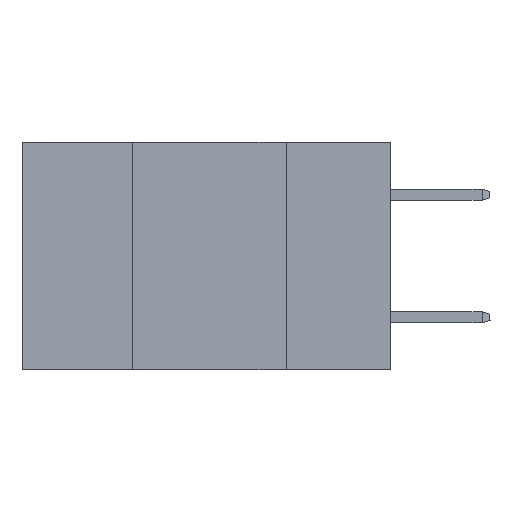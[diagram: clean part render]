
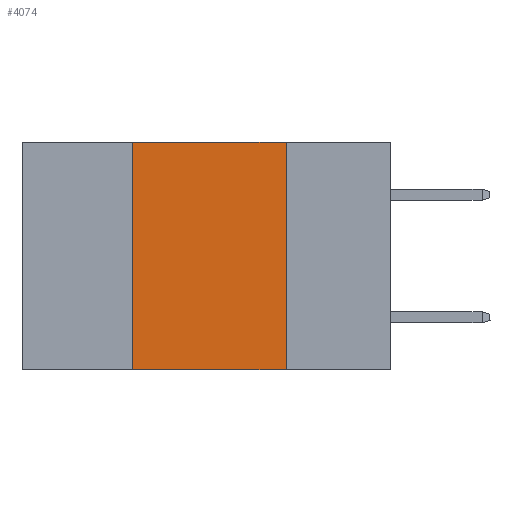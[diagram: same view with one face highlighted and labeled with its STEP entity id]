
A CAD part, left-side view. The second image highlights one B-rep face of the part: STEP entity #4074.
In plain terms, the highlighted planar face has unit normal (-1, 0, 0).
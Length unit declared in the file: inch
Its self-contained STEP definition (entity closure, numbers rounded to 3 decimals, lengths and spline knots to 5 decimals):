
#590 = EDGE_LOOP ( 'NONE', ( #1073, #13805, #1461, #7977 ) ) ;
#1073 = ORIENTED_EDGE ( 'NONE', *, *, #4192, .F. ) ;
#1370 = DIRECTION ( 'NONE',  ( 0., -1., 0. ) ) ;
#1461 = ORIENTED_EDGE ( 'NONE', *, *, #10347, .F. ) ;
#1855 = CARTESIAN_POINT ( 'NONE',  ( 0., 0.42, 0. ) ) ;
#2816 = LINE ( 'NONE', #6653, #6019 ) ;
#4020 = AXIS2_PLACEMENT_3D ( 'NONE', #13506, #14666, #7683 ) ;
#4074 = ADVANCED_FACE ( 'NONE', ( #7967 ), #5213, .F. ) ;
#4192 = EDGE_CURVE ( 'NONE', #4265, #5424, #2816, .T. ) ;
#4265 = VERTEX_POINT ( 'NONE', #5523 ) ;
#5213 = PLANE ( 'NONE',  #4020 ) ;
#5328 = CARTESIAN_POINT ( 'NONE',  ( 0., 0.42, 0. ) ) ;
#5424 = VERTEX_POINT ( 'NONE', #10269 ) ;
#5523 = CARTESIAN_POINT ( 'NONE',  ( 0., 0.17, 0. ) ) ;
#6019 = VECTOR ( 'NONE', #13711, 39.37008 ) ;
#6653 = CARTESIAN_POINT ( 'NONE',  ( 0., 0.17, 0. ) ) ;
#7033 = LINE ( 'NONE', #5328, #12939 ) ;
#7461 = CARTESIAN_POINT ( 'NONE',  ( 0., 0.6, -0.37 ) ) ;
#7626 = CARTESIAN_POINT ( 'NONE',  ( 0., 0.42, -0.37 ) ) ;
#7683 = DIRECTION ( 'NONE',  ( 0., 0., -1. ) ) ;
#7939 = EDGE_CURVE ( 'NONE', #8622, #4265, #9032, .T. ) ;
#7967 = FACE_OUTER_BOUND ( 'NONE', #590, .T. ) ;
#7977 = ORIENTED_EDGE ( 'NONE', *, *, #8871, .T. ) ;
#8214 = VECTOR ( 'NONE', #1370, 39.37008 ) ;
#8622 = VERTEX_POINT ( 'NONE', #1855 ) ;
#8871 = EDGE_CURVE ( 'NONE', #8971, #5424, #14035, .T. ) ;
#8971 = VERTEX_POINT ( 'NONE', #7626 ) ;
#8999 = DIRECTION ( 'NONE',  ( 0., 0., 1. ) ) ;
#9032 = LINE ( 'NONE', #11478, #14791 ) ;
#10269 = CARTESIAN_POINT ( 'NONE',  ( 0., 0.17, -0.37 ) ) ;
#10347 = EDGE_CURVE ( 'NONE', #8971, #8622, #7033, .T. ) ;
#11478 = CARTESIAN_POINT ( 'NONE',  ( 0., 0.6, 0. ) ) ;
#12666 = DIRECTION ( 'NONE',  ( 0., -1., 0. ) ) ;
#12939 = VECTOR ( 'NONE', #8999, 39.37008 ) ;
#13506 = CARTESIAN_POINT ( 'NONE',  ( 0., 0.6, 0. ) ) ;
#13711 = DIRECTION ( 'NONE',  ( 0., 0., -1. ) ) ;
#13805 = ORIENTED_EDGE ( 'NONE', *, *, #7939, .F. ) ;
#14035 = LINE ( 'NONE', #7461, #8214 ) ;
#14666 = DIRECTION ( 'NONE',  ( 1., 0., 0. ) ) ;
#14791 = VECTOR ( 'NONE', #12666, 39.37008 ) ;
